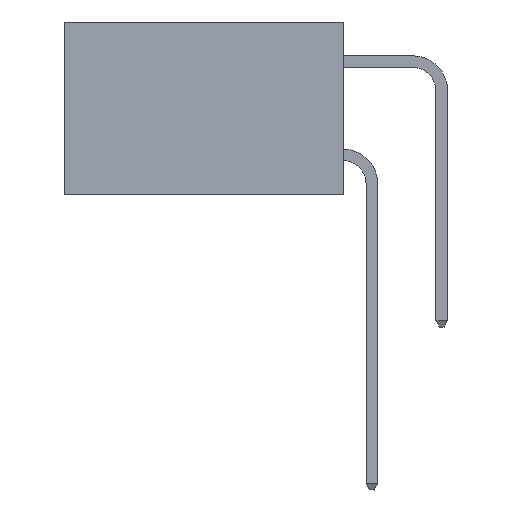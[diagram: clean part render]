
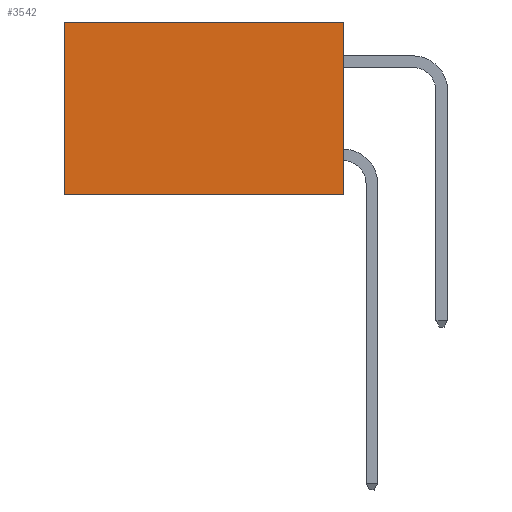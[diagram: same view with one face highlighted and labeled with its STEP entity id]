
A CAD part, left-side view. The second image highlights one B-rep face of the part: STEP entity #3542.
In plain terms, the highlighted planar face has unit normal (-1, 0, 0).
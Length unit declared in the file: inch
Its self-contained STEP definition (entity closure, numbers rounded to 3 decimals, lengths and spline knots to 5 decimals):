
#141 = ORIENTED_EDGE ( 'NONE', *, *, #2224, .F. ) ;
#152 = CARTESIAN_POINT ( 'NONE',  ( 0.298, 0.6, -0.37 ) ) ;
#402 = VECTOR ( 'NONE', #8317, 39.37008 ) ;
#506 = CARTESIAN_POINT ( 'NONE',  ( 0.298, 0., -0.37 ) ) ;
#954 = LINE ( 'NONE', #11077, #402 ) ;
#1103 = ORIENTED_EDGE ( 'NONE', *, *, #3405, .T. ) ;
#1928 = FACE_OUTER_BOUND ( 'NONE', #3626, .T. ) ;
#2224 = EDGE_CURVE ( 'NONE', #8776, #8934, #4869, .T. ) ;
#2658 = AXIS2_PLACEMENT_3D ( 'NONE', #8319, #9288, #10119 ) ;
#3027 = CARTESIAN_POINT ( 'NONE',  ( 0.298, 0., 0. ) ) ;
#3254 = VECTOR ( 'NONE', #7328, 39.37008 ) ;
#3354 = CARTESIAN_POINT ( 'NONE',  ( 0.298, 0.6, 0. ) ) ;
#3405 = EDGE_CURVE ( 'NONE', #8776, #3715, #8735, .T. ) ;
#3542 = ADVANCED_FACE ( 'NONE', ( #1928 ), #5777, .F. ) ;
#3626 = EDGE_LOOP ( 'NONE', ( #10669, #7530, #141, #1103 ) ) ;
#3715 = VERTEX_POINT ( 'NONE', #3354 ) ;
#3740 = DIRECTION ( 'NONE',  ( 0., 1., 0. ) ) ;
#4869 = LINE ( 'NONE', #11060, #6106 ) ;
#5777 = PLANE ( 'NONE',  #2658 ) ;
#6106 = VECTOR ( 'NONE', #9220, 39.37008 ) ;
#6367 = VECTOR ( 'NONE', #3740, 39.37008 ) ;
#6979 = LINE ( 'NONE', #10904, #3254 ) ;
#7211 = EDGE_CURVE ( 'NONE', #8934, #11133, #954, .T. ) ;
#7328 = DIRECTION ( 'NONE',  ( 0., 0., -1. ) ) ;
#7530 = ORIENTED_EDGE ( 'NONE', *, *, #7211, .F. ) ;
#8317 = DIRECTION ( 'NONE',  ( 0., 1., 0. ) ) ;
#8319 = CARTESIAN_POINT ( 'NONE',  ( 0.298, 0., 0. ) ) ;
#8735 = LINE ( 'NONE', #9048, #6367 ) ;
#8776 = VERTEX_POINT ( 'NONE', #3027 ) ;
#8934 = VERTEX_POINT ( 'NONE', #506 ) ;
#9048 = CARTESIAN_POINT ( 'NONE',  ( 0.298, 0., 0. ) ) ;
#9220 = DIRECTION ( 'NONE',  ( 0., 0., -1. ) ) ;
#9288 = DIRECTION ( 'NONE',  ( 1., 0., 0. ) ) ;
#10119 = DIRECTION ( 'NONE',  ( 0., 0., -1. ) ) ;
#10669 = ORIENTED_EDGE ( 'NONE', *, *, #10797, .T. ) ;
#10797 = EDGE_CURVE ( 'NONE', #3715, #11133, #6979, .T. ) ;
#10904 = CARTESIAN_POINT ( 'NONE',  ( 0.298, 0.6, 0. ) ) ;
#11060 = CARTESIAN_POINT ( 'NONE',  ( 0.298, 0., 0. ) ) ;
#11077 = CARTESIAN_POINT ( 'NONE',  ( 0.298, 0., -0.37 ) ) ;
#11133 = VERTEX_POINT ( 'NONE', #152 ) ;
